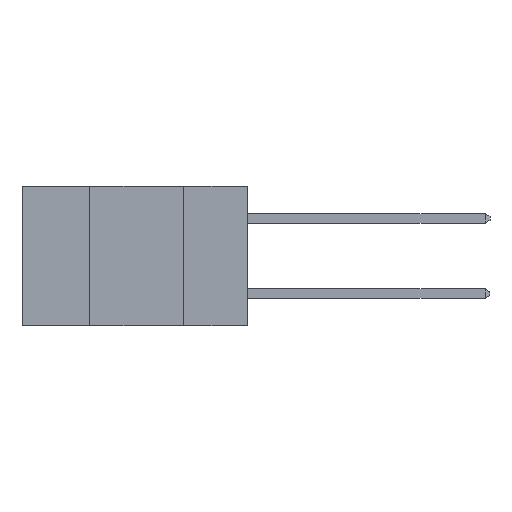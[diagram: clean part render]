
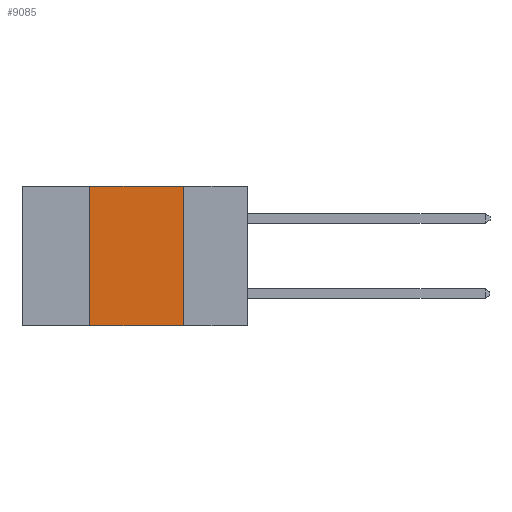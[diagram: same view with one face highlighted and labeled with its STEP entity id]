
A CAD part, left-side view. The second image highlights one B-rep face of the part: STEP entity #9085.
In plain terms, the highlighted planar face has unit normal (-1, 0, 0).
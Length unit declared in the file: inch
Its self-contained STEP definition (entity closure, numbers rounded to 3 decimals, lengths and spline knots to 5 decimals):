
#772 = VERTEX_POINT ( 'NONE', #13567 ) ;
#1148 = DIRECTION ( 'NONE',  ( 0., 0., -1. ) ) ;
#1325 = EDGE_LOOP ( 'NONE', ( #13038, #8779, #9529, #2958 ) ) ;
#2523 = DIRECTION ( 'NONE',  ( 0., -1., 0. ) ) ;
#2602 = LINE ( 'NONE', #8459, #9626 ) ;
#2958 = ORIENTED_EDGE ( 'NONE', *, *, #9231, .T. ) ;
#2959 = CARTESIAN_POINT ( 'NONE',  ( 0., 0.6, -0.37 ) ) ;
#3586 = EDGE_CURVE ( 'NONE', #4533, #11311, #2602, .T. ) ;
#4324 = CARTESIAN_POINT ( 'NONE',  ( 0., 0.17, 0. ) ) ;
#4533 = VERTEX_POINT ( 'NONE', #4324 ) ;
#6582 = FACE_OUTER_BOUND ( 'NONE', #1325, .T. ) ;
#6634 = DIRECTION ( 'NONE',  ( 1., 0., 0. ) ) ;
#6694 = CARTESIAN_POINT ( 'NONE',  ( 0., 0.6, 0. ) ) ;
#8287 = EDGE_CURVE ( 'NONE', #772, #12400, #9923, .T. ) ;
#8323 = DIRECTION ( 'NONE',  ( 0., 0., 1. ) ) ;
#8459 = CARTESIAN_POINT ( 'NONE',  ( 0., 0.17, 0. ) ) ;
#8779 = ORIENTED_EDGE ( 'NONE', *, *, #15712, .F. ) ;
#9085 = ADVANCED_FACE ( 'NONE', ( #6582 ), #14925, .F. ) ;
#9231 = EDGE_CURVE ( 'NONE', #772, #11311, #12256, .T. ) ;
#9529 = ORIENTED_EDGE ( 'NONE', *, *, #8287, .F. ) ;
#9626 = VECTOR ( 'NONE', #1148, 39.37008 ) ;
#9923 = LINE ( 'NONE', #13546, #13140 ) ;
#10024 = CARTESIAN_POINT ( 'NONE',  ( 0., 0.17, -0.37 ) ) ;
#11311 = VERTEX_POINT ( 'NONE', #10024 ) ;
#11827 = VECTOR ( 'NONE', #12726, 39.37008 ) ;
#12256 = LINE ( 'NONE', #2959, #11827 ) ;
#12400 = VERTEX_POINT ( 'NONE', #15492 ) ;
#12726 = DIRECTION ( 'NONE',  ( 0., -1., 0. ) ) ;
#13038 = ORIENTED_EDGE ( 'NONE', *, *, #3586, .F. ) ;
#13140 = VECTOR ( 'NONE', #8323, 39.37008 ) ;
#13546 = CARTESIAN_POINT ( 'NONE',  ( 0., 0.42, 0. ) ) ;
#13567 = CARTESIAN_POINT ( 'NONE',  ( 0., 0.42, -0.37 ) ) ;
#13577 = CARTESIAN_POINT ( 'NONE',  ( 0., 0.6, 0. ) ) ;
#13883 = AXIS2_PLACEMENT_3D ( 'NONE', #13577, #6634, #16304 ) ;
#14359 = LINE ( 'NONE', #6694, #17481 ) ;
#14925 = PLANE ( 'NONE',  #13883 ) ;
#15492 = CARTESIAN_POINT ( 'NONE',  ( 0., 0.42, 0. ) ) ;
#15712 = EDGE_CURVE ( 'NONE', #12400, #4533, #14359, .T. ) ;
#16304 = DIRECTION ( 'NONE',  ( 0., 0., -1. ) ) ;
#17481 = VECTOR ( 'NONE', #2523, 39.37008 ) ;
